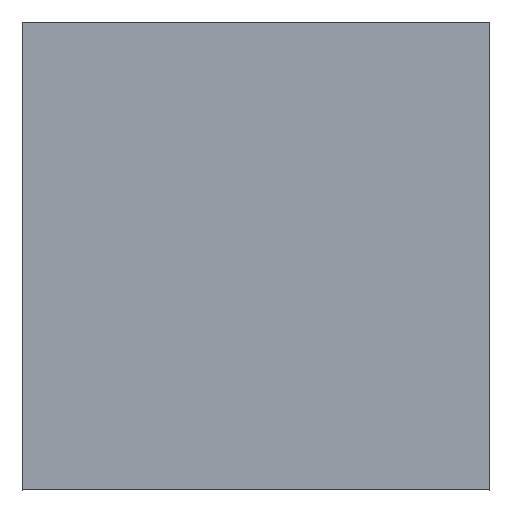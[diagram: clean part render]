
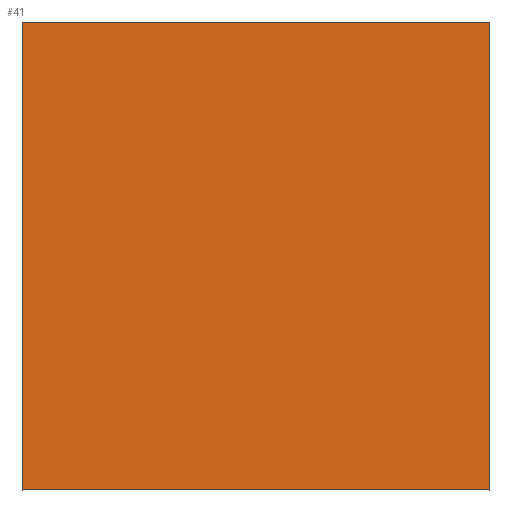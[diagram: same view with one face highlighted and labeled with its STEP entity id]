
A CAD part, top view. The second image highlights one B-rep face of the part: STEP entity #41.
In plain terms, the highlighted planar face has unit normal (0, 0, 1).
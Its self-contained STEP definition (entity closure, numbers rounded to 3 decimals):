
#14 = CARTESIAN_POINT ( 'NONE',  ( -5., 5., 4.2 ) ) ;
#19 = CARTESIAN_POINT ( 'NONE',  ( -5., 5., 4.2 ) ) ;
#41 = ADVANCED_FACE ( 'NONE', ( #106 ), #174, .F. ) ;
#57 = VERTEX_POINT ( 'NONE', #175 ) ;
#71 = VECTOR ( 'NONE', #443, 1000. ) ;
#73 = VERTEX_POINT ( 'NONE', #394 ) ;
#81 = VECTOR ( 'NONE', #189, 1000. ) ;
#87 = VERTEX_POINT ( 'NONE', #211 ) ;
#95 = EDGE_LOOP ( 'NONE', ( #380, #450, #300, #367 ) ) ;
#106 = FACE_OUTER_BOUND ( 'NONE', #95, .T. ) ;
#111 = EDGE_CURVE ( 'NONE', #73, #87, #346, .T. ) ;
#119 = CARTESIAN_POINT ( 'NONE',  ( -5., 5., 4.2 ) ) ;
#144 = DIRECTION ( 'NONE',  ( -1., 0., 0. ) ) ;
#174 = PLANE ( 'NONE',  #276 ) ;
#175 = CARTESIAN_POINT ( 'NONE',  ( 5., 5., 4.2 ) ) ;
#189 = DIRECTION ( 'NONE',  ( 1., 0., 0. ) ) ;
#205 = VERTEX_POINT ( 'NONE', #119 ) ;
#211 = CARTESIAN_POINT ( 'NONE',  ( 5., -5., 4.2 ) ) ;
#224 = LINE ( 'NONE', #19, #230 ) ;
#230 = VECTOR ( 'NONE', #298, 1000. ) ;
#240 = EDGE_CURVE ( 'NONE', #205, #57, #279, .T. ) ;
#247 = DIRECTION ( 'NONE',  ( 1., 0., 0. ) ) ;
#250 = EDGE_CURVE ( 'NONE', #205, #73, #224, .T. ) ;
#258 = VECTOR ( 'NONE', #247, 1000. ) ;
#268 = EDGE_CURVE ( 'NONE', #57, #87, #405, .T. ) ;
#276 = AXIS2_PLACEMENT_3D ( 'NONE', #321, #361, #144 ) ;
#279 = LINE ( 'NONE', #14, #81 ) ;
#298 = DIRECTION ( 'NONE',  ( 0., -1., 0. ) ) ;
#300 = ORIENTED_EDGE ( 'NONE', *, *, #111, .T. ) ;
#321 = CARTESIAN_POINT ( 'NONE',  ( 0., 0., 4.2 ) ) ;
#346 = LINE ( 'NONE', #436, #258 ) ;
#361 = DIRECTION ( 'NONE',  ( 0., 0., -1. ) ) ;
#367 = ORIENTED_EDGE ( 'NONE', *, *, #268, .F. ) ;
#380 = ORIENTED_EDGE ( 'NONE', *, *, #240, .F. ) ;
#383 = CARTESIAN_POINT ( 'NONE',  ( 5., 5., 4.2 ) ) ;
#394 = CARTESIAN_POINT ( 'NONE',  ( -5., -5., 4.2 ) ) ;
#405 = LINE ( 'NONE', #383, #71 ) ;
#436 = CARTESIAN_POINT ( 'NONE',  ( -5., -5., 4.2 ) ) ;
#443 = DIRECTION ( 'NONE',  ( 0., -1., 0. ) ) ;
#450 = ORIENTED_EDGE ( 'NONE', *, *, #250, .T. ) ;
